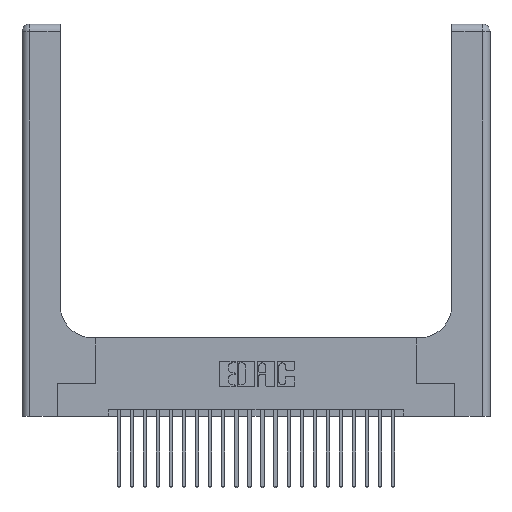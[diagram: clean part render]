
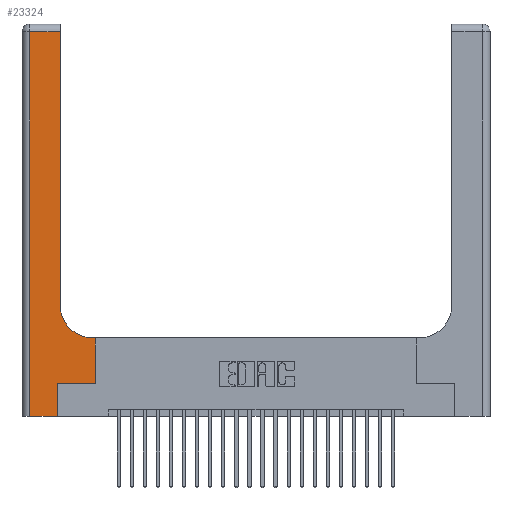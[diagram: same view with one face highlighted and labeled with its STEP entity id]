
A CAD part, top view. The second image highlights one B-rep face of the part: STEP entity #23324.
In plain terms, the highlighted planar face has unit normal (0, 0, 1).
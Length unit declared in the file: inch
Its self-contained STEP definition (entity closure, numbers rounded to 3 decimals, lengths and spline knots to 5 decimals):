
#671 = LINE ( 'NONE', #1176, #15929 ) ;
#1176 = CARTESIAN_POINT ( 'NONE',  ( 0., 2.94, 0.37 ) ) ;
#1742 = CARTESIAN_POINT ( 'NONE',  ( 0.06, 3., 0.37 ) ) ;
#1750 = CARTESIAN_POINT ( 'NONE',  ( 0.5585, 0.25, 0.37 ) ) ;
#1878 = PLANE ( 'NONE',  #11864 ) ;
#2200 = CARTESIAN_POINT ( 'NONE',  ( 0.2915, 0.6, 0.37 ) ) ;
#2892 = ORIENTED_EDGE ( 'NONE', *, *, #24290, .T. ) ;
#2973 = DIRECTION ( 'NONE',  ( 0., 0., -1. ) ) ;
#3825 = LINE ( 'NONE', #1742, #24755 ) ;
#3826 = EDGE_CURVE ( 'NONE', #12655, #15741, #14101, .T. ) ;
#4285 = CARTESIAN_POINT ( 'NONE',  ( 0.5585, 0.6, 0.37 ) ) ;
#4818 = LINE ( 'NONE', #9192, #23014 ) ;
#4960 = CARTESIAN_POINT ( 'NONE',  ( 0.06, 0., 0.37 ) ) ;
#5016 = EDGE_CURVE ( 'NONE', #23190, #6616, #15588, .T. ) ;
#5166 = CARTESIAN_POINT ( 'NONE',  ( 0.2915, 3., 0.37 ) ) ;
#5407 = DIRECTION ( 'NONE',  ( 0., 1., 0. ) ) ;
#5436 = VERTEX_POINT ( 'NONE', #17368 ) ;
#5723 = DIRECTION ( 'NONE',  ( 0., -1., 0. ) ) ;
#5760 = LINE ( 'NONE', #15526, #24275 ) ;
#5778 = DIRECTION ( 'NONE',  ( 1., 0., 0. ) ) ;
#6541 = CIRCLE ( 'NONE', #12517, 0.25 ) ;
#6616 = VERTEX_POINT ( 'NONE', #22987 ) ;
#7264 = VERTEX_POINT ( 'NONE', #13468 ) ;
#7741 = CARTESIAN_POINT ( 'NONE',  ( 0.269, 0., 0.37 ) ) ;
#8918 = EDGE_CURVE ( 'NONE', #19268, #7264, #11905, .T. ) ;
#9084 = CARTESIAN_POINT ( 'NONE',  ( 0.269, 0.25, 0.37 ) ) ;
#9192 = CARTESIAN_POINT ( 'NONE',  ( 0.269, 0., 0.37 ) ) ;
#9402 = FACE_OUTER_BOUND ( 'NONE', #15226, .T. ) ;
#9916 = LINE ( 'NONE', #1750, #20517 ) ;
#10549 = DIRECTION ( 'NONE',  ( 1., 0., 0. ) ) ;
#10815 = EDGE_CURVE ( 'NONE', #15741, #25118, #4818, .T. ) ;
#10905 = ORIENTED_EDGE ( 'NONE', *, *, #8918, .T. ) ;
#11428 = CARTESIAN_POINT ( 'NONE',  ( 0., 3., 0.37 ) ) ;
#11594 = EDGE_CURVE ( 'NONE', #5436, #19268, #9916, .T. ) ;
#11864 = AXIS2_PLACEMENT_3D ( 'NONE', #11428, #17482, #25091 ) ;
#11905 = LINE ( 'NONE', #2200, #19801 ) ;
#11919 = VECTOR ( 'NONE', #16856, 39.37008 ) ;
#12169 = EDGE_CURVE ( 'NONE', #13014, #12655, #3825, .T. ) ;
#12517 = AXIS2_PLACEMENT_3D ( 'NONE', #20217, #2973, #10549 ) ;
#12655 = VERTEX_POINT ( 'NONE', #4960 ) ;
#12660 = ORIENTED_EDGE ( 'NONE', *, *, #10815, .T. ) ;
#12793 = EDGE_CURVE ( 'NONE', #7264, #23190, #6541, .T. ) ;
#13014 = VERTEX_POINT ( 'NONE', #21253 ) ;
#13086 = DIRECTION ( 'NONE',  ( -1., 0., 0. ) ) ;
#13468 = CARTESIAN_POINT ( 'NONE',  ( 0.5415, 0.6, 0.37 ) ) ;
#13520 = DIRECTION ( 'NONE',  ( 0., 1., 0. ) ) ;
#14101 = LINE ( 'NONE', #19323, #16225 ) ;
#14861 = ORIENTED_EDGE ( 'NONE', *, *, #11594, .T. ) ;
#15152 = ORIENTED_EDGE ( 'NONE', *, *, #16597, .T. ) ;
#15226 = EDGE_LOOP ( 'NONE', ( #16956, #15152, #15275, #18430, #12660, #2892, #14861, #10905, #17453 ) ) ;
#15275 = ORIENTED_EDGE ( 'NONE', *, *, #12169, .T. ) ;
#15526 = CARTESIAN_POINT ( 'NONE',  ( 0.269, 0.25, 0.37 ) ) ;
#15588 = LINE ( 'NONE', #5166, #11919 ) ;
#15741 = VERTEX_POINT ( 'NONE', #7741 ) ;
#15929 = VECTOR ( 'NONE', #13086, 39.37008 ) ;
#16225 = VECTOR ( 'NONE', #5778, 39.37008 ) ;
#16597 = EDGE_CURVE ( 'NONE', #6616, #13014, #671, .T. ) ;
#16856 = DIRECTION ( 'NONE',  ( 0., 1., 0. ) ) ;
#16956 = ORIENTED_EDGE ( 'NONE', *, *, #5016, .T. ) ;
#17368 = CARTESIAN_POINT ( 'NONE',  ( 0.5585, 0.25, 0.37 ) ) ;
#17453 = ORIENTED_EDGE ( 'NONE', *, *, #12793, .T. ) ;
#17482 = DIRECTION ( 'NONE',  ( 0., 0., -1. ) ) ;
#18430 = ORIENTED_EDGE ( 'NONE', *, *, #3826, .T. ) ;
#19268 = VERTEX_POINT ( 'NONE', #4285 ) ;
#19323 = CARTESIAN_POINT ( 'NONE',  ( 0., 0., 0.37 ) ) ;
#19641 = DIRECTION ( 'NONE',  ( -1., 0., 0. ) ) ;
#19759 = DIRECTION ( 'NONE',  ( 1., 0., 0. ) ) ;
#19801 = VECTOR ( 'NONE', #19641, 39.37008 ) ;
#20217 = CARTESIAN_POINT ( 'NONE',  ( 0.5415, 0.85, 0.37 ) ) ;
#20517 = VECTOR ( 'NONE', #13520, 39.37008 ) ;
#21253 = CARTESIAN_POINT ( 'NONE',  ( 0.06, 2.94, 0.37 ) ) ;
#22987 = CARTESIAN_POINT ( 'NONE',  ( 0.2915, 2.94, 0.37 ) ) ;
#23014 = VECTOR ( 'NONE', #5407, 39.37008 ) ;
#23190 = VERTEX_POINT ( 'NONE', #24660 ) ;
#23324 = ADVANCED_FACE ( 'NONE', ( #9402 ), #1878, .F. ) ;
#24275 = VECTOR ( 'NONE', #19759, 39.37008 ) ;
#24290 = EDGE_CURVE ( 'NONE', #25118, #5436, #5760, .T. ) ;
#24660 = CARTESIAN_POINT ( 'NONE',  ( 0.2915, 0.85, 0.37 ) ) ;
#24755 = VECTOR ( 'NONE', #5723, 39.37008 ) ;
#25091 = DIRECTION ( 'NONE',  ( -1., 0., 0. ) ) ;
#25118 = VERTEX_POINT ( 'NONE', #9084 ) ;
